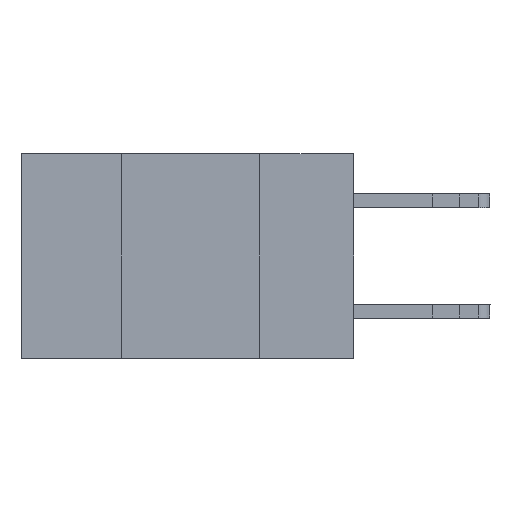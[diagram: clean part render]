
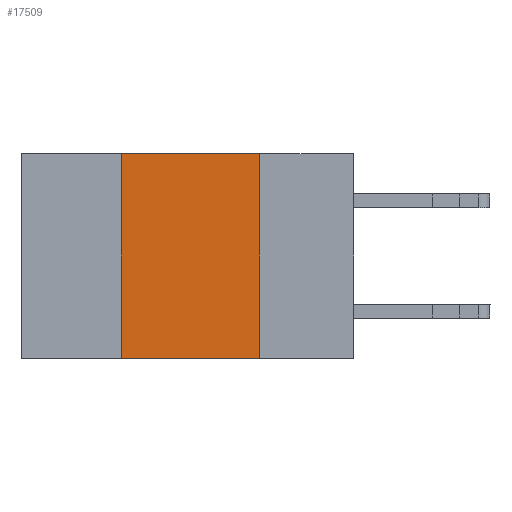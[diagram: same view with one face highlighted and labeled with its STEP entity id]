
A CAD part, left-side view. The second image highlights one B-rep face of the part: STEP entity #17509.
In plain terms, the highlighted planar face has unit normal (-1, 0, 0).
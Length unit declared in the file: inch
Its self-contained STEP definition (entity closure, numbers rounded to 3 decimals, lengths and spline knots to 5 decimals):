
#31 = VERTEX_POINT ( 'NONE', #7481 ) ;
#751 = PLANE ( 'NONE',  #17746 ) ;
#1452 = CARTESIAN_POINT ( 'NONE',  ( 0., 0.42, 0. ) ) ;
#2289 = ORIENTED_EDGE ( 'NONE', *, *, #4084, .T. ) ;
#2896 = LINE ( 'NONE', #9370, #12856 ) ;
#3052 = ORIENTED_EDGE ( 'NONE', *, *, #23684, .F. ) ;
#3532 = EDGE_LOOP ( 'NONE', ( #24316, #16186, #3052, #2289 ) ) ;
#4084 = EDGE_CURVE ( 'NONE', #16021, #31, #18729, .T. ) ;
#4214 = VECTOR ( 'NONE', #9120, 39.37008 ) ;
#6722 = LINE ( 'NONE', #20183, #14194 ) ;
#7481 = CARTESIAN_POINT ( 'NONE',  ( 0., 0.17, -0.37 ) ) ;
#8834 = LINE ( 'NONE', #17598, #4214 ) ;
#9120 = DIRECTION ( 'NONE',  ( 0., 0., -1. ) ) ;
#9370 = CARTESIAN_POINT ( 'NONE',  ( 0., 0.6, 0. ) ) ;
#12856 = VECTOR ( 'NONE', #16420, 39.37008 ) ;
#13707 = EDGE_CURVE ( 'NONE', #15248, #20725, #2896, .T. ) ;
#14194 = VECTOR ( 'NONE', #26658, 39.37008 ) ;
#14251 = CARTESIAN_POINT ( 'NONE',  ( 0., 0.6, 0. ) ) ;
#14390 = DIRECTION ( 'NONE',  ( 0., 0., -1. ) ) ;
#15248 = VERTEX_POINT ( 'NONE', #1452 ) ;
#16021 = VERTEX_POINT ( 'NONE', #20354 ) ;
#16186 = ORIENTED_EDGE ( 'NONE', *, *, #13707, .F. ) ;
#16420 = DIRECTION ( 'NONE',  ( 0., -1., 0. ) ) ;
#16586 = CARTESIAN_POINT ( 'NONE',  ( 0., 0.6, -0.37 ) ) ;
#16693 = FACE_OUTER_BOUND ( 'NONE', #3532, .T. ) ;
#17509 = ADVANCED_FACE ( 'NONE', ( #16693 ), #751, .F. ) ;
#17598 = CARTESIAN_POINT ( 'NONE',  ( 0., 0.17, 0. ) ) ;
#17746 = AXIS2_PLACEMENT_3D ( 'NONE', #14251, #18276, #14390 ) ;
#18276 = DIRECTION ( 'NONE',  ( 1., 0., 0. ) ) ;
#18528 = EDGE_CURVE ( 'NONE', #20725, #31, #8834, .T. ) ;
#18729 = LINE ( 'NONE', #16586, #24049 ) ;
#20183 = CARTESIAN_POINT ( 'NONE',  ( 0., 0.42, 0. ) ) ;
#20354 = CARTESIAN_POINT ( 'NONE',  ( 0., 0.42, -0.37 ) ) ;
#20725 = VERTEX_POINT ( 'NONE', #25462 ) ;
#23684 = EDGE_CURVE ( 'NONE', #16021, #15248, #6722, .T. ) ;
#24049 = VECTOR ( 'NONE', #27488, 39.37008 ) ;
#24316 = ORIENTED_EDGE ( 'NONE', *, *, #18528, .F. ) ;
#25462 = CARTESIAN_POINT ( 'NONE',  ( 0., 0.17, 0. ) ) ;
#26658 = DIRECTION ( 'NONE',  ( 0., 0., 1. ) ) ;
#27488 = DIRECTION ( 'NONE',  ( 0., -1., 0. ) ) ;
